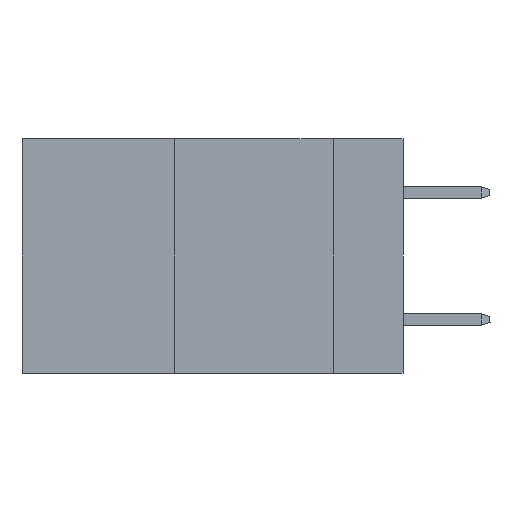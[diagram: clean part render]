
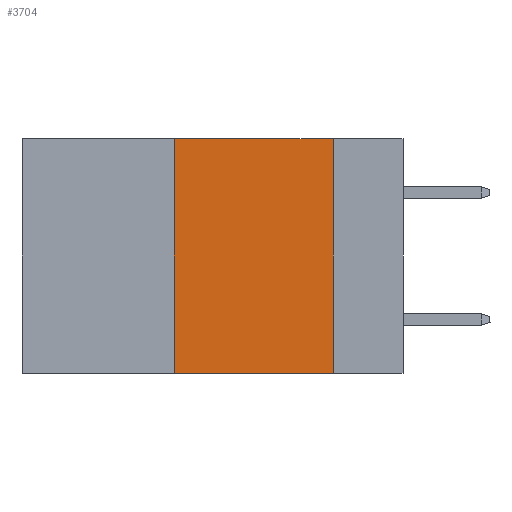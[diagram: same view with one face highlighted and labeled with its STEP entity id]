
A CAD part, left-side view. The second image highlights one B-rep face of the part: STEP entity #3704.
In plain terms, the highlighted planar face has unit normal (-1, 0, 0).
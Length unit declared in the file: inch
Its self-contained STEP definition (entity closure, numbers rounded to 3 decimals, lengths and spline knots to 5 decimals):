
#131 = CARTESIAN_POINT ( 'NONE',  ( 0., 0.11, 0. ) ) ;
#211 = CARTESIAN_POINT ( 'NONE',  ( 0., 0.36, 0. ) ) ;
#384 = DIRECTION ( 'NONE',  ( 0., -1., 0. ) ) ;
#1164 = DIRECTION ( 'NONE',  ( 0., 0., -1. ) ) ;
#1595 = EDGE_CURVE ( 'NONE', #18753, #9911, #18190, .T. ) ;
#2774 = LINE ( 'NONE', #9387, #21591 ) ;
#3003 = DIRECTION ( 'NONE',  ( 0., 0., -1. ) ) ;
#3210 = EDGE_LOOP ( 'NONE', ( #18771, #6631, #12568, #21247 ) ) ;
#3298 = DIRECTION ( 'NONE',  ( 0., -1., 0. ) ) ;
#3704 = ADVANCED_FACE ( 'NONE', ( #11398 ), #16570, .F. ) ;
#4370 = CARTESIAN_POINT ( 'NONE',  ( 0., 0.36, -0.37 ) ) ;
#5692 = CARTESIAN_POINT ( 'NONE',  ( 0., 0.11, -0.37 ) ) ;
#6631 = ORIENTED_EDGE ( 'NONE', *, *, #15715, .F. ) ;
#8596 = VECTOR ( 'NONE', #1164, 39.37008 ) ;
#9387 = CARTESIAN_POINT ( 'NONE',  ( 0., 0.36, 0. ) ) ;
#9911 = VERTEX_POINT ( 'NONE', #5692 ) ;
#11367 = CARTESIAN_POINT ( 'NONE',  ( 0., 0.6, -0.37 ) ) ;
#11398 = FACE_OUTER_BOUND ( 'NONE', #3210, .T. ) ;
#12568 = ORIENTED_EDGE ( 'NONE', *, *, #16414, .F. ) ;
#12844 = LINE ( 'NONE', #11367, #18377 ) ;
#13164 = VERTEX_POINT ( 'NONE', #4370 ) ;
#15114 = VECTOR ( 'NONE', #384, 39.37008 ) ;
#15437 = AXIS2_PLACEMENT_3D ( 'NONE', #21734, #18351, #3003 ) ;
#15715 = EDGE_CURVE ( 'NONE', #16247, #18753, #19091, .T. ) ;
#16247 = VERTEX_POINT ( 'NONE', #211 ) ;
#16414 = EDGE_CURVE ( 'NONE', #13164, #16247, #2774, .T. ) ;
#16570 = PLANE ( 'NONE',  #15437 ) ;
#16911 = EDGE_CURVE ( 'NONE', #13164, #9911, #12844, .T. ) ;
#17205 = CARTESIAN_POINT ( 'NONE',  ( 0., 0.6, 0. ) ) ;
#18190 = LINE ( 'NONE', #18411, #8596 ) ;
#18351 = DIRECTION ( 'NONE',  ( 1., 0., 0. ) ) ;
#18377 = VECTOR ( 'NONE', #3298, 39.37008 ) ;
#18411 = CARTESIAN_POINT ( 'NONE',  ( 0., 0.11, 0. ) ) ;
#18753 = VERTEX_POINT ( 'NONE', #131 ) ;
#18771 = ORIENTED_EDGE ( 'NONE', *, *, #1595, .F. ) ;
#19091 = LINE ( 'NONE', #17205, #15114 ) ;
#21171 = DIRECTION ( 'NONE',  ( 0., 0., 1. ) ) ;
#21247 = ORIENTED_EDGE ( 'NONE', *, *, #16911, .T. ) ;
#21591 = VECTOR ( 'NONE', #21171, 39.37008 ) ;
#21734 = CARTESIAN_POINT ( 'NONE',  ( 0., 0.6, 0. ) ) ;
